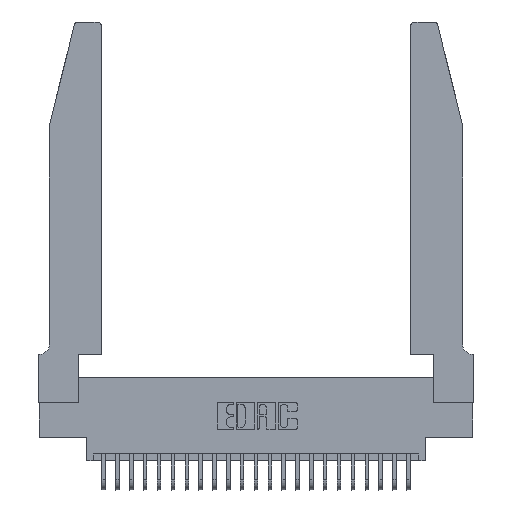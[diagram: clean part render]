
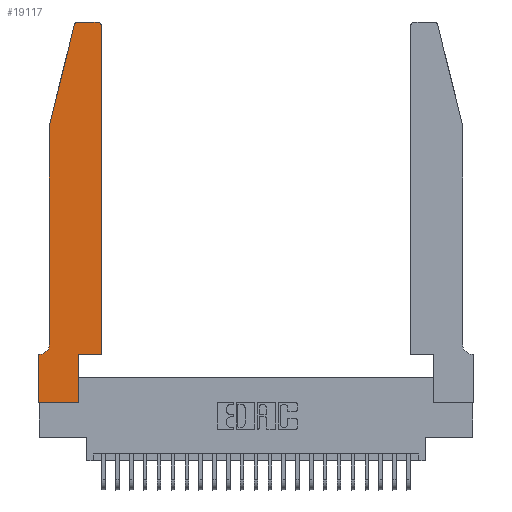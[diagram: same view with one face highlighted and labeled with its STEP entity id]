
A CAD part, top view. The second image highlights one B-rep face of the part: STEP entity #19117.
In plain terms, the highlighted planar face has unit normal (0, 0, 1).
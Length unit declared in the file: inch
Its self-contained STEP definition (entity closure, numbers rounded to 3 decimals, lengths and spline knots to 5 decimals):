
#80 = CARTESIAN_POINT ( 'NONE',  ( 0.25487, 2.72718, 0.37 ) ) ;
#306 = EDGE_CURVE ( 'NONE', #21819, #16718, #16291, .T. ) ;
#395 = VECTOR ( 'NONE', #12045, 39.37008 ) ;
#1559 = CARTESIAN_POINT ( 'NONE',  ( 0., 0., 0.37 ) ) ;
#1674 = VERTEX_POINT ( 'NONE', #1559 ) ;
#1780 = EDGE_CURVE ( 'NONE', #20225, #6853, #13183, .T. ) ;
#2085 = VERTEX_POINT ( 'NONE', #18255 ) ;
#2476 = ORIENTED_EDGE ( 'NONE', *, *, #14703, .T. ) ;
#3045 = AXIS2_PLACEMENT_3D ( 'NONE', #20614, #16565, #18683 ) ;
#3111 = VERTEX_POINT ( 'NONE', #10459 ) ;
#3191 = EDGE_CURVE ( 'NONE', #2085, #1674, #7581, .T. ) ;
#3623 = CARTESIAN_POINT ( 'NONE',  ( 0.0755, 2., 0.37 ) ) ;
#3890 = AXIS2_PLACEMENT_3D ( 'NONE', #6158, #6067, #4295 ) ;
#3918 = CARTESIAN_POINT ( 'NONE',  ( 0.0755, 0.35, 0.37 ) ) ;
#3955 = DIRECTION ( 'NONE',  ( 1., 0., 0. ) ) ;
#4295 = DIRECTION ( 'NONE',  ( -1., 0., 0. ) ) ;
#4334 = EDGE_CURVE ( 'NONE', #3111, #21819, #10758, .T. ) ;
#4654 = CARTESIAN_POINT ( 'NONE',  ( 0.0755, 0.42, 0.37 ) ) ;
#4839 = CARTESIAN_POINT ( 'NONE',  ( 0.0755, 2., 0.37 ) ) ;
#4878 = DIRECTION ( 'NONE',  ( 0., -1., 0. ) ) ;
#5202 = EDGE_LOOP ( 'NONE', ( #2476, #15562, #20264, #22823, #12336, #9790, #25089, #24636, #19984, #14604, #13410, #7395 ) ) ;
#6067 = DIRECTION ( 'NONE',  ( 0., 0., -1. ) ) ;
#6158 = CARTESIAN_POINT ( 'NONE',  ( 0.0055, 0.42, 0.37 ) ) ;
#6654 = CARTESIAN_POINT ( 'NONE',  ( 0.4505, 0.35, 0.37 ) ) ;
#6853 = VERTEX_POINT ( 'NONE', #4839 ) ;
#6986 = CIRCLE ( 'NONE', #3045, 0.03 ) ;
#7250 = VERTEX_POINT ( 'NONE', #4654 ) ;
#7395 = ORIENTED_EDGE ( 'NONE', *, *, #306, .T. ) ;
#7581 = LINE ( 'NONE', #23199, #19374 ) ;
#7778 = CARTESIAN_POINT ( 'NONE',  ( 0.4505, 0.35, 0.37 ) ) ;
#8026 = VECTOR ( 'NONE', #3955, 39.37008 ) ;
#8464 = EDGE_CURVE ( 'NONE', #23324, #20225, #6986, .T. ) ;
#8475 = EDGE_CURVE ( 'NONE', #25167, #2085, #26365, .T. ) ;
#8731 = EDGE_CURVE ( 'NONE', #6853, #7250, #22066, .T. ) ;
#8953 = FACE_OUTER_BOUND ( 'NONE', #5202, .T. ) ;
#9790 = ORIENTED_EDGE ( 'NONE', *, *, #8475, .T. ) ;
#10064 = DIRECTION ( 'NONE',  ( -1., 0., 0. ) ) ;
#10332 = EDGE_CURVE ( 'NONE', #11673, #3111, #19421, .T. ) ;
#10459 = CARTESIAN_POINT ( 'NONE',  ( 0.4505, 0.35, 0.37 ) ) ;
#10758 = LINE ( 'NONE', #7778, #15674 ) ;
#10783 = CARTESIAN_POINT ( 'NONE',  ( 0.2865, 0.35, 0.37 ) ) ;
#10828 = CARTESIAN_POINT ( 'NONE',  ( 0.284, 2.75, 0.37 ) ) ;
#11673 = VERTEX_POINT ( 'NONE', #18836 ) ;
#12045 = DIRECTION ( 'NONE',  ( -0.239, -0.971, 0. ) ) ;
#12054 = CARTESIAN_POINT ( 'NONE',  ( 0.2865, 0., 0.37 ) ) ;
#12121 = CARTESIAN_POINT ( 'NONE',  ( 0.4205, 2.72, 0.37 ) ) ;
#12296 = CARTESIAN_POINT ( 'NONE',  ( 0., 0., 0.37 ) ) ;
#12336 = ORIENTED_EDGE ( 'NONE', *, *, #24682, .T. ) ;
#12506 = VECTOR ( 'NONE', #20803, 39.37008 ) ;
#12702 = DIRECTION ( 'NONE',  ( -1., 0., 0. ) ) ;
#12711 = DIRECTION ( 'NONE',  ( 0., 1., 0. ) ) ;
#12754 = VECTOR ( 'NONE', #12702, 39.37008 ) ;
#13183 = LINE ( 'NONE', #3623, #395 ) ;
#13197 = DIRECTION ( 'NONE',  ( 0., -1., 0. ) ) ;
#13410 = ORIENTED_EDGE ( 'NONE', *, *, #4334, .T. ) ;
#13737 = CARTESIAN_POINT ( 'NONE',  ( 0.0055, 0.35, 0.37 ) ) ;
#14132 = DIRECTION ( 'NONE',  ( 1., 0., 0. ) ) ;
#14380 = AXIS2_PLACEMENT_3D ( 'NONE', #12121, #20390, #14132 ) ;
#14487 = VECTOR ( 'NONE', #4878, 39.37008 ) ;
#14604 = ORIENTED_EDGE ( 'NONE', *, *, #10332, .T. ) ;
#14657 = EDGE_CURVE ( 'NONE', #25932, #11673, #20659, .T. ) ;
#14703 = EDGE_CURVE ( 'NONE', #16718, #23324, #24603, .T. ) ;
#14897 = CARTESIAN_POINT ( 'NONE',  ( 0.4505, 2.72, 0.37 ) ) ;
#15314 = CARTESIAN_POINT ( 'NONE',  ( 0., 0.35, 0.37 ) ) ;
#15562 = ORIENTED_EDGE ( 'NONE', *, *, #8464, .T. ) ;
#15674 = VECTOR ( 'NONE', #22431, 39.37008 ) ;
#16081 = AXIS2_PLACEMENT_3D ( 'NONE', #15314, #21222, #23532 ) ;
#16291 = CIRCLE ( 'NONE', #14380, 0.03 ) ;
#16565 = DIRECTION ( 'NONE',  ( 0., 0., 1. ) ) ;
#16718 = VERTEX_POINT ( 'NONE', #26013 ) ;
#16988 = CARTESIAN_POINT ( 'NONE',  ( 0.0755, 2., 0.37 ) ) ;
#18255 = CARTESIAN_POINT ( 'NONE',  ( 0., 0.35, 0.37 ) ) ;
#18683 = DIRECTION ( 'NONE',  ( 1., 0., 0. ) ) ;
#18836 = CARTESIAN_POINT ( 'NONE',  ( 0.2865, 0.35, 0.37 ) ) ;
#19117 = ADVANCED_FACE ( 'NONE', ( #8953 ), #25539, .T. ) ;
#19374 = VECTOR ( 'NONE', #13197, 39.37008 ) ;
#19421 = LINE ( 'NONE', #6654, #12506 ) ;
#19984 = ORIENTED_EDGE ( 'NONE', *, *, #14657, .T. ) ;
#20157 = LINE ( 'NONE', #12296, #8026 ) ;
#20225 = VERTEX_POINT ( 'NONE', #80 ) ;
#20264 = ORIENTED_EDGE ( 'NONE', *, *, #1780, .T. ) ;
#20390 = DIRECTION ( 'NONE',  ( 0., 0., 1. ) ) ;
#20614 = CARTESIAN_POINT ( 'NONE',  ( 0.284, 2.72, 0.37 ) ) ;
#20659 = LINE ( 'NONE', #10783, #24916 ) ;
#20803 = DIRECTION ( 'NONE',  ( 1., 0., 0. ) ) ;
#21222 = DIRECTION ( 'NONE',  ( 0., 0., 1. ) ) ;
#21819 = VERTEX_POINT ( 'NONE', #14897 ) ;
#22066 = LINE ( 'NONE', #16988, #14487 ) ;
#22415 = VECTOR ( 'NONE', #10064, 39.37008 ) ;
#22431 = DIRECTION ( 'NONE',  ( 0., 1., 0. ) ) ;
#22823 = ORIENTED_EDGE ( 'NONE', *, *, #8731, .T. ) ;
#23199 = CARTESIAN_POINT ( 'NONE',  ( 0., 0., 0.37 ) ) ;
#23324 = VERTEX_POINT ( 'NONE', #10828 ) ;
#23532 = DIRECTION ( 'NONE',  ( 1., 0., 0. ) ) ;
#24091 = CIRCLE ( 'NONE', #3890, 0.07 ) ;
#24603 = LINE ( 'NONE', #25276, #12754 ) ;
#24636 = ORIENTED_EDGE ( 'NONE', *, *, #24715, .T. ) ;
#24682 = EDGE_CURVE ( 'NONE', #7250, #25167, #24091, .T. ) ;
#24715 = EDGE_CURVE ( 'NONE', #1674, #25932, #20157, .T. ) ;
#24916 = VECTOR ( 'NONE', #12711, 39.37008 ) ;
#25089 = ORIENTED_EDGE ( 'NONE', *, *, #3191, .T. ) ;
#25167 = VERTEX_POINT ( 'NONE', #13737 ) ;
#25276 = CARTESIAN_POINT ( 'NONE',  ( 0.2605, 2.75, 0.37 ) ) ;
#25539 = PLANE ( 'NONE',  #16081 ) ;
#25932 = VERTEX_POINT ( 'NONE', #12054 ) ;
#26013 = CARTESIAN_POINT ( 'NONE',  ( 0.4205, 2.75, 0.37 ) ) ;
#26365 = LINE ( 'NONE', #3918, #22415 ) ;
